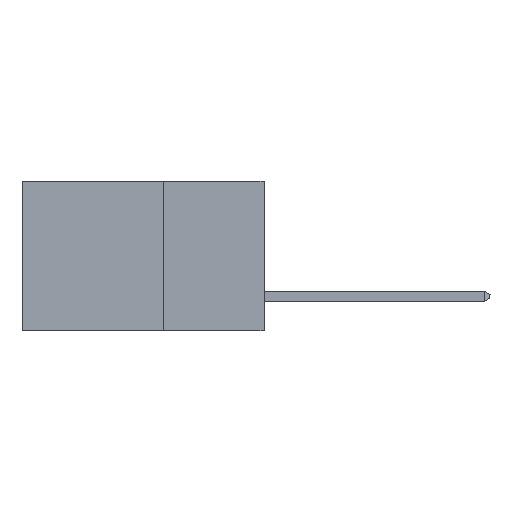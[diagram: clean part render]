
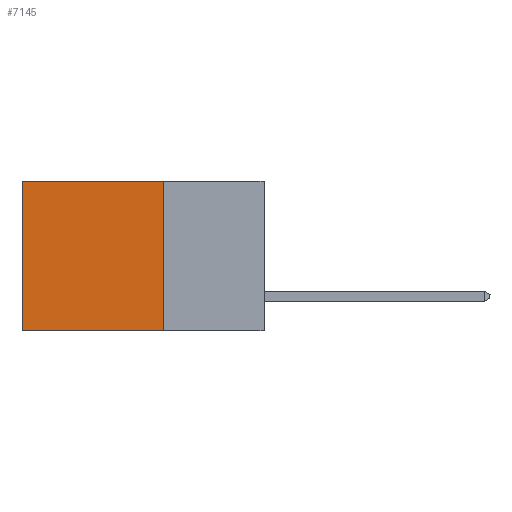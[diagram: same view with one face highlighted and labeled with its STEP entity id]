
A CAD part, left-side view. The second image highlights one B-rep face of the part: STEP entity #7145.
In plain terms, the highlighted planar face has unit normal (-1, 0, 0).
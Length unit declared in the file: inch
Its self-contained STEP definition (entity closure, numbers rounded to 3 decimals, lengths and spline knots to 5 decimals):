
#1496 = PLANE ( 'NONE',  #6807 ) ;
#1578 = VERTEX_POINT ( 'NONE', #14513 ) ;
#1929 = EDGE_CURVE ( 'NONE', #1578, #4825, #12249, .T. ) ;
#2372 = VERTEX_POINT ( 'NONE', #7298 ) ;
#2857 = DIRECTION ( 'NONE',  ( 0., 1., 0. ) ) ;
#2893 = LINE ( 'NONE', #12426, #3407 ) ;
#3339 = EDGE_CURVE ( 'NONE', #2372, #12683, #2893, .T. ) ;
#3407 = VECTOR ( 'NONE', #14740, 39.37008 ) ;
#3665 = CARTESIAN_POINT ( 'NONE',  ( 0.2615, 0.25, -0.37 ) ) ;
#3700 = DIRECTION ( 'NONE',  ( 0., 0., -1. ) ) ;
#3743 = DIRECTION ( 'NONE',  ( 0., 0., -1. ) ) ;
#4825 = VERTEX_POINT ( 'NONE', #8347 ) ;
#4957 = CARTESIAN_POINT ( 'NONE',  ( 0.2615, 0.25, -0.37 ) ) ;
#5955 = ORIENTED_EDGE ( 'NONE', *, *, #1929, .F. ) ;
#6138 = VECTOR ( 'NONE', #8489, 39.37008 ) ;
#6178 = EDGE_CURVE ( 'NONE', #1578, #2372, #8558, .T. ) ;
#6324 = ORIENTED_EDGE ( 'NONE', *, *, #9957, .F. ) ;
#6807 = AXIS2_PLACEMENT_3D ( 'NONE', #4957, #14588, #3700 ) ;
#7145 = ADVANCED_FACE ( 'NONE', ( #11182 ), #1496, .F. ) ;
#7298 = CARTESIAN_POINT ( 'NONE',  ( 0.2615, 0.6, 0. ) ) ;
#8347 = CARTESIAN_POINT ( 'NONE',  ( 0.2615, 0.25, -0.37 ) ) ;
#8489 = DIRECTION ( 'NONE',  ( 0., 1., 0. ) ) ;
#8558 = LINE ( 'NONE', #13346, #14099 ) ;
#8901 = EDGE_LOOP ( 'NONE', ( #10928, #6324, #5955, #10753 ) ) ;
#9108 = CARTESIAN_POINT ( 'NONE',  ( 0.2615, 0.6, -0.37 ) ) ;
#9674 = LINE ( 'NONE', #3665, #6138 ) ;
#9957 = EDGE_CURVE ( 'NONE', #4825, #12683, #9674, .T. ) ;
#10753 = ORIENTED_EDGE ( 'NONE', *, *, #6178, .T. ) ;
#10928 = ORIENTED_EDGE ( 'NONE', *, *, #3339, .T. ) ;
#11182 = FACE_OUTER_BOUND ( 'NONE', #8901, .T. ) ;
#12249 = LINE ( 'NONE', #13001, #12673 ) ;
#12426 = CARTESIAN_POINT ( 'NONE',  ( 0.2615, 0.6, -0.37 ) ) ;
#12673 = VECTOR ( 'NONE', #3743, 39.37008 ) ;
#12683 = VERTEX_POINT ( 'NONE', #9108 ) ;
#13001 = CARTESIAN_POINT ( 'NONE',  ( 0.2615, 0.25, -0.37 ) ) ;
#13346 = CARTESIAN_POINT ( 'NONE',  ( 0.2615, 0.25, 0. ) ) ;
#14099 = VECTOR ( 'NONE', #2857, 39.37008 ) ;
#14513 = CARTESIAN_POINT ( 'NONE',  ( 0.2615, 0.25, 0. ) ) ;
#14588 = DIRECTION ( 'NONE',  ( 1., 0., 0. ) ) ;
#14740 = DIRECTION ( 'NONE',  ( 0., 0., -1. ) ) ;
